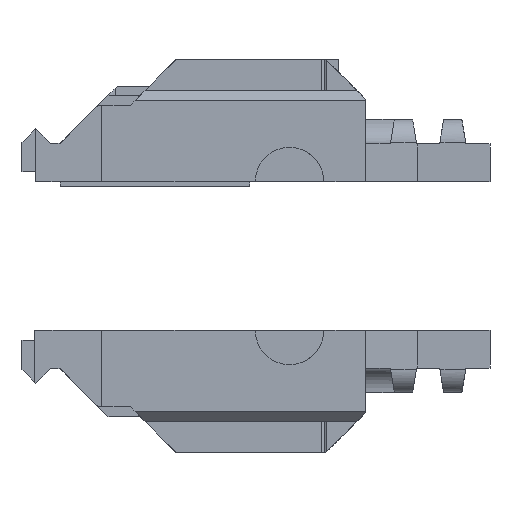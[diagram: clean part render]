
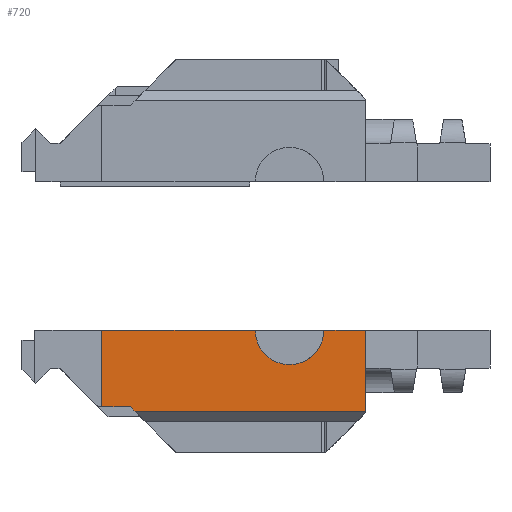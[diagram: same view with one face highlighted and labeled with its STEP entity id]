
A CAD part, left-side view. The second image highlights one B-rep face of the part: STEP entity #720.
In plain terms, the highlighted planar face has unit normal (-1, 0, 0).
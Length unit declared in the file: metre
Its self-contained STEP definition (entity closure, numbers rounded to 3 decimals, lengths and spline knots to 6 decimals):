
#720=ADVANCED_FACE('0:1553',(#2882),#2883,.F.);
#2882=FACE_OUTER_BOUND('',#6254,.T.);
#2883=PLANE('',#6255);
#6254=EDGE_LOOP('',(#12991,#12992,#12993,#12994,#12995,#12996,#12997,#12998,#12999));
#6255=AXIS2_PLACEMENT_3D('',#13000,#13001,#13002);
#12991=ORIENTED_EDGE('',*,*,#24382,.F.);
#12992=ORIENTED_EDGE('',*,*,#24830,.T.);
#12993=ORIENTED_EDGE('',*,*,#24831,.F.);
#12994=ORIENTED_EDGE('',*,*,#24832,.T.);
#12995=ORIENTED_EDGE('',*,*,#23036,.F.);
#12996=ORIENTED_EDGE('',*,*,#23138,.F.);
#12997=ORIENTED_EDGE('',*,*,#24833,.T.);
#12998=ORIENTED_EDGE('',*,*,#24536,.T.);
#12999=ORIENTED_EDGE('',*,*,#24768,.F.);
#13000=CARTESIAN_POINT('',(-0.203,0.0,0.0));
#13001=DIRECTION('',(1.0,0.0,-0.0));
#13002=DIRECTION('',(-0.0,1.0,0.0));
#23036=EDGE_CURVE('0:2521',#27645,#27648,#27649,.T.);
#23138=EDGE_CURVE('0:2521',#27831,#27645,#27833,.T.);
#24382=EDGE_CURVE('0:6322',#29992,#29994,#29995,.T.);
#24536=EDGE_CURVE('0:6889',#30259,#30256,#30260,.T.);
#24768=EDGE_CURVE('0:7585',#29994,#30256,#30657,.T.);
#24830=EDGE_CURVE('0:7771',#29992,#30749,#30751,.T.);
#24831=EDGE_CURVE('0:7774',#30752,#30749,#30753,.T.);
#24832=EDGE_CURVE('0:7777',#30752,#27648,#30754,.T.);
#24833=EDGE_CURVE('0:7780',#27831,#30259,#30755,.T.);
#27645=VERTEX_POINT('',#35294);
#27648=VERTEX_POINT('NONE',#35298);
#27649=CIRCLE('',#35299,0.006875);
#27831=VERTEX_POINT('NONE',#35583);
#27833=CIRCLE('',#35586,0.006875);
#29992=VERTEX_POINT('NONE',#39351);
#29994=VERTEX_POINT('NONE',#39354);
#29995=LINE('',#39355,#39356);
#30256=VERTEX_POINT('NONE',#39738);
#30259=VERTEX_POINT('NONE',#39742);
#30260=LINE('',#39743,#39744);
#30657=LINE('',#40371,#40372);
#30749=VERTEX_POINT('NONE',#40517);
#30751=LINE('',#40520,#40521);
#30752=VERTEX_POINT('NONE',#40522);
#30753=LINE('',#40523,#40524);
#30754=LINE('',#40525,#40526);
#30755=LINE('',#40527,#40528);
#35294=CARTESIAN_POINT('',(-0.203,0.01524,-0.006875));
#35298=CARTESIAN_POINT('',(-0.203,0.008365,0.0));
#35299=AXIS2_PLACEMENT_3D('',#49054,#49055,#49056);
#35583=CARTESIAN_POINT('',(-0.203,0.022115,0.0));
#35586=AXIS2_PLACEMENT_3D('',#49217,#49218,#49219);
#39351=CARTESIAN_POINT('',(-0.203,0.046263,-0.016238));
#39354=CARTESIAN_POINT('',(-0.203,0.047197,-0.015304));
#39355=CARTESIAN_POINT('',(-0.203,0.04,-0.0225));
#39356=VECTOR('',#50683,1.0);
#39738=CARTESIAN_POINT('',(-0.203,0.052959,-0.015304));
#39742=CARTESIAN_POINT('',(-0.203,0.052959,0.0));
#39743=CARTESIAN_POINT('',(-0.203,0.052959,0.0));
#39744=VECTOR('',#50899,1.0);
#40371=CARTESIAN_POINT('',(-0.203,0.047197,-0.015304));
#40372=VECTOR('',#51133,1.0);
#40517=CARTESIAN_POINT('',(-0.203,0.,-0.016238));
#40520=CARTESIAN_POINT('',(-0.203,0.0,-0.016238));
#40521=VECTOR('',#51209,1.0);
#40522=CARTESIAN_POINT('',(-0.203,0.0,0.0));
#40523=CARTESIAN_POINT('',(-0.203,0.0,0.0));
#40524=VECTOR('',#51210,1.0);
#40525=CARTESIAN_POINT('',(-0.203,0.0,0.0));
#40526=VECTOR('',#51211,1.0);
#40527=CARTESIAN_POINT('',(-0.203,0.0,0.0));
#40528=VECTOR('',#51212,1.0);
#49054=CARTESIAN_POINT('',(-0.203,0.01524,0.0));
#49055=DIRECTION('',(-1.0,0.0,0.0));
#49056=DIRECTION('',(0.0,0.0,1.0));
#49217=CARTESIAN_POINT('',(-0.203,0.01524,0.0));
#49218=DIRECTION('',(-1.0,0.0,0.0));
#49219=DIRECTION('',(0.0,0.0,1.0));
#50683=DIRECTION('',(0.0,0.707,0.707));
#50899=DIRECTION('',(0.0,0.0,-1.0));
#51133=DIRECTION('',(0.0,1.0,0.));
#51209=DIRECTION('',(0.0,-1.0,0.0));
#51210=DIRECTION('',(0.0,0.,-1.0));
#51211=DIRECTION('',(0.0,1.0,0.0));
#51212=DIRECTION('',(0.0,1.0,0.0));
